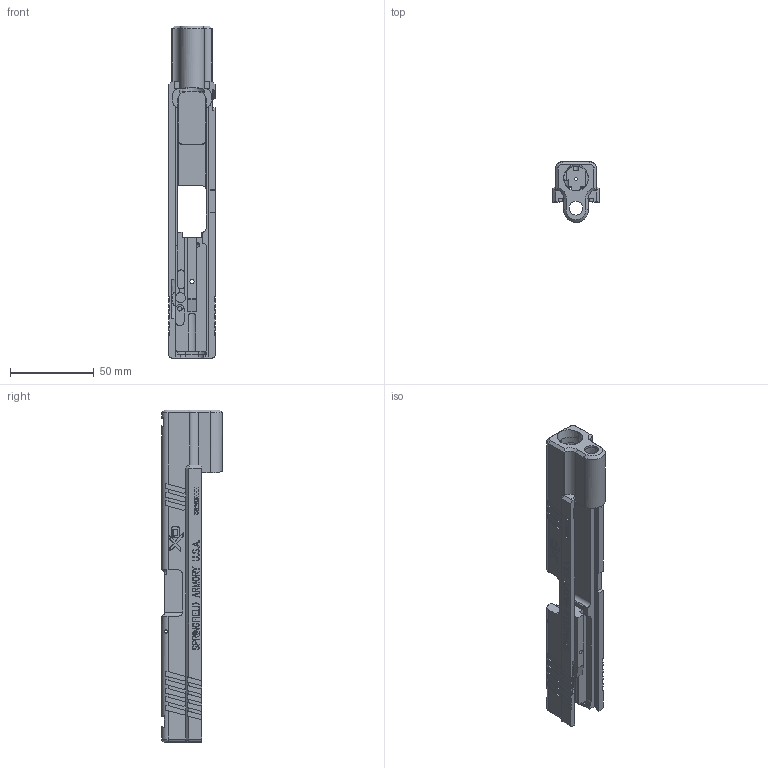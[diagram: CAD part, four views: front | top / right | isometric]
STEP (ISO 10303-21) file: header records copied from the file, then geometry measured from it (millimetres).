
FILE_DESCRIPTION (( 'STEP AP214' ), '1' );
FILE_NAME ('SLIDE - XD-40 Tactical.STEP', '2013-06-19T13:59:18', ( 'Asher' ), ( '' ), 'SwSTEP 2.0', 'SolidWorks 2013', '' );
FILE_SCHEMA (( 'AUTOMOTIVE_DESIGN' ));
Length unit declared in the file: millimetre
Products named in the file (1): SLIDE - XD-40 Tactical
Bounding box: 27.69 x 36.27 x 198.44 mm (x, y, z)
Volume: 52702.7 mm3; surface area: 32810.3 mm2
Topology: 1 solids, 1 shells, 3042 faces, 8618 edges, 5727 vertices
Faces by surface type: plane 2018, bspline 678, cylinder 329, cone 11, torus 6
Entity records: 110622 total; most frequent: CARTESIAN_POINT 35901, ORIENTED_EDGE 17236, DIRECTION 12534, EDGE_CURVE 8618, LINE 6478, VECTOR 6478, VERTEX_POINT 5727, EDGE_LOOP 3217
